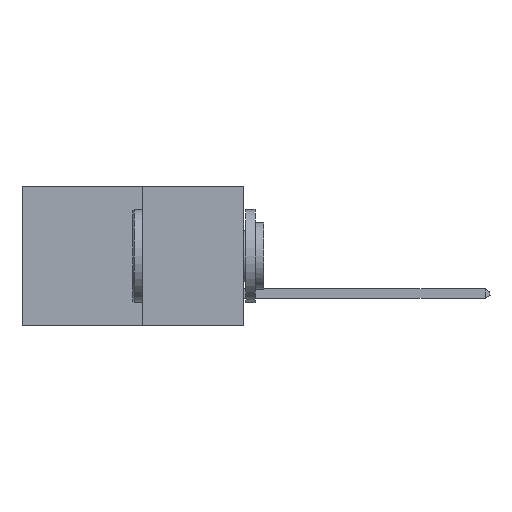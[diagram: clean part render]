
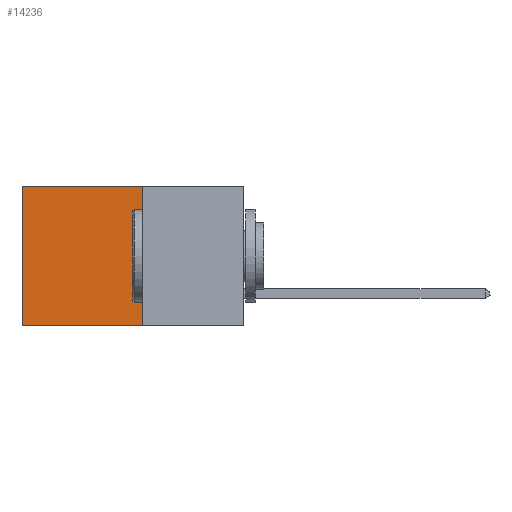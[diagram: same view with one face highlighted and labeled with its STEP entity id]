
A CAD part, left-side view. The second image highlights one B-rep face of the part: STEP entity #14236.
In plain terms, the highlighted planar face has unit normal (-1, 0, 0).
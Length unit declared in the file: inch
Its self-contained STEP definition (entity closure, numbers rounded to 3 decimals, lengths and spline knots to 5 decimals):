
#184 = ORIENTED_EDGE ( 'NONE', *, *, #18911, .F. ) ;
#1666 = DIRECTION ( 'NONE',  ( 1., 0., 0. ) ) ;
#2375 = DIRECTION ( 'NONE',  ( 0., 0., -1. ) ) ;
#5180 = CARTESIAN_POINT ( 'NONE',  ( 0.277, 0.27, 0. ) ) ;
#5530 = VERTEX_POINT ( 'NONE', #15683 ) ;
#5676 = VERTEX_POINT ( 'NONE', #12672 ) ;
#5714 = CARTESIAN_POINT ( 'NONE',  ( 0.277, 0.27, -0.37 ) ) ;
#6189 = AXIS2_PLACEMENT_3D ( 'NONE', #9992, #1666, #13346 ) ;
#6660 = CARTESIAN_POINT ( 'NONE',  ( 0.277, 0.59, -0.37 ) ) ;
#6953 = LINE ( 'NONE', #6660, #20104 ) ;
#7277 = CARTESIAN_POINT ( 'NONE',  ( 0.277, 0.27, 0. ) ) ;
#7393 = DIRECTION ( 'NONE',  ( 0., 1., 0. ) ) ;
#7839 = LINE ( 'NONE', #5714, #16138 ) ;
#7912 = EDGE_LOOP ( 'NONE', ( #18550, #11144, #184, #10680 ) ) ;
#8589 = EDGE_CURVE ( 'NONE', #18862, #13235, #11904, .T. ) ;
#9095 = CARTESIAN_POINT ( 'NONE',  ( 0.277, 0.59, 0. ) ) ;
#9474 = DIRECTION ( 'NONE',  ( 0., 0., -1. ) ) ;
#9992 = CARTESIAN_POINT ( 'NONE',  ( 0.277, 0.27, -0.37 ) ) ;
#10680 = ORIENTED_EDGE ( 'NONE', *, *, #8589, .T. ) ;
#11144 = ORIENTED_EDGE ( 'NONE', *, *, #16443, .F. ) ;
#11672 = PLANE ( 'NONE',  #6189 ) ;
#11904 = LINE ( 'NONE', #5180, #16281 ) ;
#12672 = CARTESIAN_POINT ( 'NONE',  ( 0.277, 0.59, -0.37 ) ) ;
#12956 = LINE ( 'NONE', #15701, #16810 ) ;
#13235 = VERTEX_POINT ( 'NONE', #9095 ) ;
#13346 = DIRECTION ( 'NONE',  ( 0., 0., -1. ) ) ;
#13627 = EDGE_CURVE ( 'NONE', #13235, #5676, #6953, .T. ) ;
#14236 = ADVANCED_FACE ( 'NONE', ( #21032 ), #11672, .F. ) ;
#15142 = DIRECTION ( 'NONE',  ( 0., 1., 0. ) ) ;
#15683 = CARTESIAN_POINT ( 'NONE',  ( 0.277, 0.27, -0.37 ) ) ;
#15701 = CARTESIAN_POINT ( 'NONE',  ( 0.277, 0.27, -0.37 ) ) ;
#16138 = VECTOR ( 'NONE', #7393, 39.37008 ) ;
#16281 = VECTOR ( 'NONE', #15142, 39.37008 ) ;
#16443 = EDGE_CURVE ( 'NONE', #5530, #5676, #7839, .T. ) ;
#16810 = VECTOR ( 'NONE', #2375, 39.37008 ) ;
#18550 = ORIENTED_EDGE ( 'NONE', *, *, #13627, .T. ) ;
#18862 = VERTEX_POINT ( 'NONE', #7277 ) ;
#18911 = EDGE_CURVE ( 'NONE', #18862, #5530, #12956, .T. ) ;
#20104 = VECTOR ( 'NONE', #9474, 39.37008 ) ;
#21032 = FACE_OUTER_BOUND ( 'NONE', #7912, .T. ) ;
